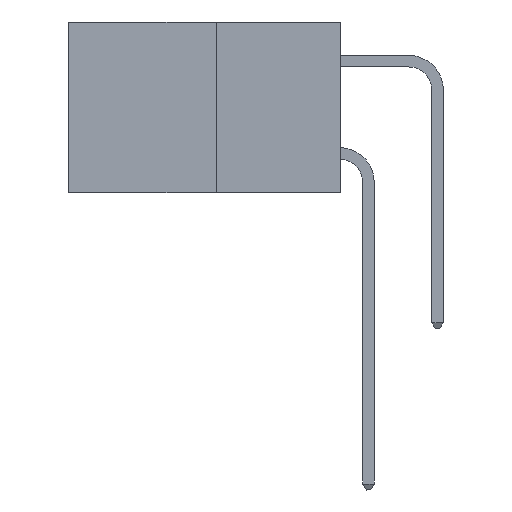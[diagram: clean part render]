
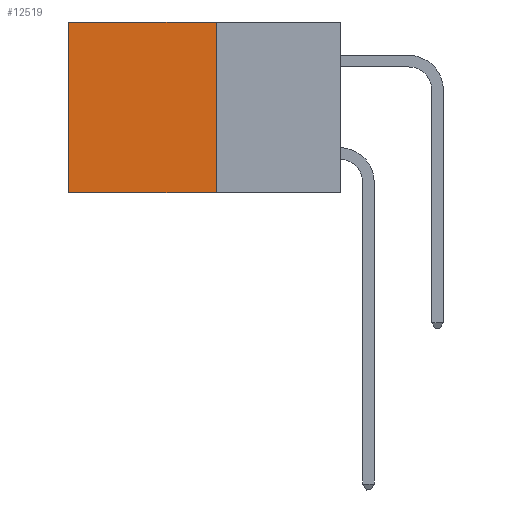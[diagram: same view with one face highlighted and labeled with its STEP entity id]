
A CAD part, left-side view. The second image highlights one B-rep face of the part: STEP entity #12519.
In plain terms, the highlighted planar face has unit normal (-1, 0, 0).
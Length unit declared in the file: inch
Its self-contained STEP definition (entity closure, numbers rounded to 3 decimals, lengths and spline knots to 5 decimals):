
#134 = DIRECTION ( 'NONE',  ( 0., 0., -1. ) ) ;
#811 = CARTESIAN_POINT ( 'NONE',  ( 0.277, 0.27, -0.37 ) ) ;
#1456 = LINE ( 'NONE', #13284, #23511 ) ;
#1743 = VERTEX_POINT ( 'NONE', #13781 ) ;
#2047 = LINE ( 'NONE', #21148, #11234 ) ;
#2427 = LINE ( 'NONE', #811, #21332 ) ;
#2846 = DIRECTION ( 'NONE',  ( 1., 0., 0. ) ) ;
#3646 = VERTEX_POINT ( 'NONE', #14597 ) ;
#5200 = VECTOR ( 'NONE', #7288, 39.37008 ) ;
#5793 = LINE ( 'NONE', #21919, #5200 ) ;
#7288 = DIRECTION ( 'NONE',  ( 0., 0., -1. ) ) ;
#7546 = EDGE_CURVE ( 'NONE', #8916, #3646, #2427, .T. ) ;
#8864 = ORIENTED_EDGE ( 'NONE', *, *, #7546, .F. ) ;
#8916 = VERTEX_POINT ( 'NONE', #9217 ) ;
#8964 = ORIENTED_EDGE ( 'NONE', *, *, #13195, .T. ) ;
#9217 = CARTESIAN_POINT ( 'NONE',  ( 0.277, 0.27, 0. ) ) ;
#9711 = DIRECTION ( 'NONE',  ( 0., 1., 0. ) ) ;
#10392 = EDGE_CURVE ( 'NONE', #3646, #10855, #1456, .T. ) ;
#10855 = VERTEX_POINT ( 'NONE', #15977 ) ;
#11234 = VECTOR ( 'NONE', #19293, 39.37008 ) ;
#11967 = CARTESIAN_POINT ( 'NONE',  ( 0.277, 0.27, -0.37 ) ) ;
#12294 = ORIENTED_EDGE ( 'NONE', *, *, #10392, .F. ) ;
#12519 = ADVANCED_FACE ( 'NONE', ( #20367 ), #13816, .F. ) ;
#13195 = EDGE_CURVE ( 'NONE', #8916, #1743, #2047, .T. ) ;
#13284 = CARTESIAN_POINT ( 'NONE',  ( 0.277, 0.27, -0.37 ) ) ;
#13781 = CARTESIAN_POINT ( 'NONE',  ( 0.277, 0.59, 0. ) ) ;
#13816 = PLANE ( 'NONE',  #18828 ) ;
#14593 = EDGE_LOOP ( 'NONE', ( #23580, #12294, #8864, #8964 ) ) ;
#14597 = CARTESIAN_POINT ( 'NONE',  ( 0.277, 0.27, -0.37 ) ) ;
#15659 = DIRECTION ( 'NONE',  ( 0., 0., -1. ) ) ;
#15977 = CARTESIAN_POINT ( 'NONE',  ( 0.277, 0.59, -0.37 ) ) ;
#18828 = AXIS2_PLACEMENT_3D ( 'NONE', #11967, #2846, #15659 ) ;
#19293 = DIRECTION ( 'NONE',  ( 0., 1., 0. ) ) ;
#20367 = FACE_OUTER_BOUND ( 'NONE', #14593, .T. ) ;
#21148 = CARTESIAN_POINT ( 'NONE',  ( 0.277, 0.27, 0. ) ) ;
#21332 = VECTOR ( 'NONE', #134, 39.37008 ) ;
#21333 = EDGE_CURVE ( 'NONE', #1743, #10855, #5793, .T. ) ;
#21919 = CARTESIAN_POINT ( 'NONE',  ( 0.277, 0.59, -0.37 ) ) ;
#23511 = VECTOR ( 'NONE', #9711, 39.37008 ) ;
#23580 = ORIENTED_EDGE ( 'NONE', *, *, #21333, .T. ) ;
